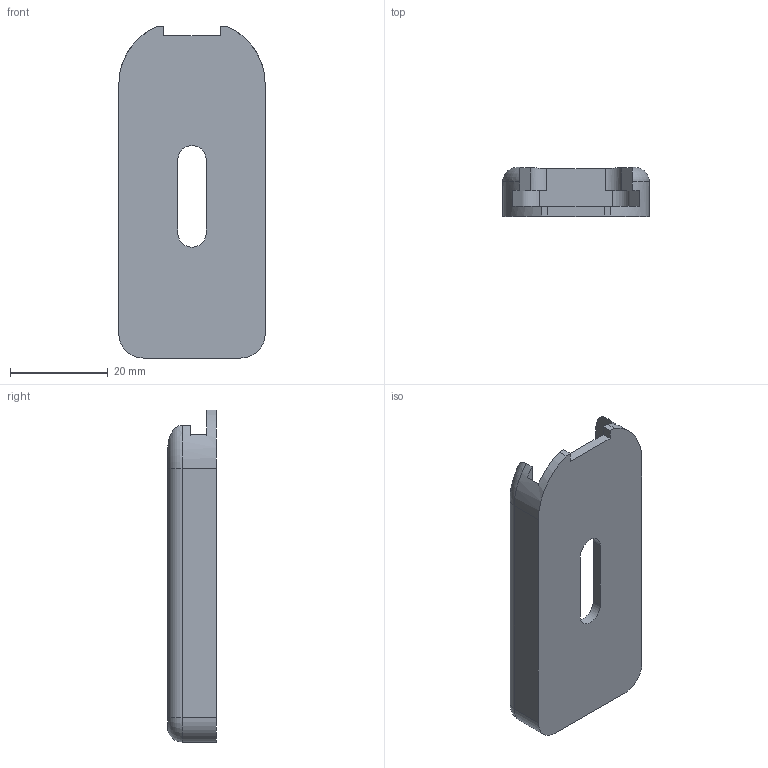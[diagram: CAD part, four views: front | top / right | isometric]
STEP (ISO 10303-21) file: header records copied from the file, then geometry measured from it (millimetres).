
FILE_DESCRIPTION (( 'STEP AP214' ), '1' );
FILE_NAME ('PmagM2Base.STEP', '2020-02-26T02:10:36', ( '' ), ( '' ), 'SwSTEP 2.0', 'SolidWorks 2019', '' );
FILE_SCHEMA (( 'AUTOMOTIVE_DESIGN' ));
Length unit declared in the file: millimetre
Products named in the file (1): PmagM2Base
Bounding box: 30 x 10 x 68 mm (x, y, z)
Volume: 6853.2 mm3; surface area: 6689.9 mm2
Topology: 1 solids, 1 shells, 43 faces, 117 edges, 76 vertices
Faces by surface type: plane 25, cylinder 14, torus 4
Entity records: 1443 total; most frequent: CARTESIAN_POINT 291, DIRECTION 237, ORIENTED_EDGE 234, EDGE_CURVE 117, AXIS2_PLACEMENT_3D 80, LINE 77, VECTOR 77, VERTEX_POINT 76
